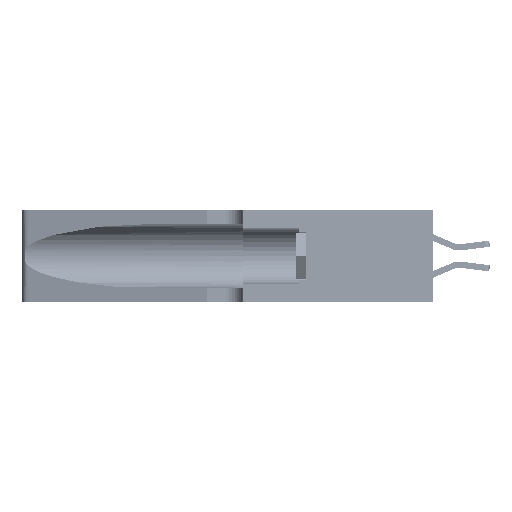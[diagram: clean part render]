
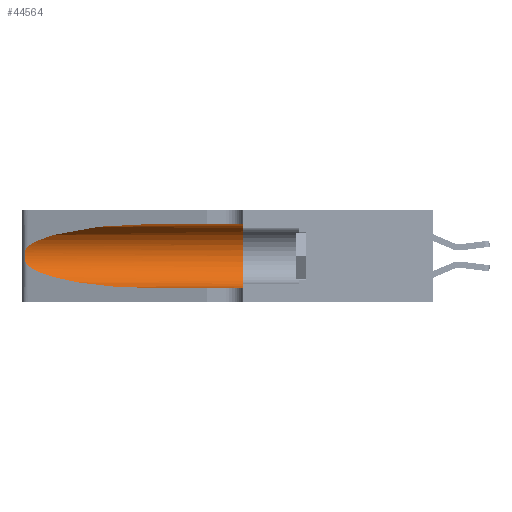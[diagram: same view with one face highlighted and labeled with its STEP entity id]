
A CAD part, left-side view. The second image highlights one B-rep face of the part: STEP entity #44564.
In plain terms, the highlighted cylindrical face has radius 3.308 mm (diameter 6.617 mm), a partial arc.
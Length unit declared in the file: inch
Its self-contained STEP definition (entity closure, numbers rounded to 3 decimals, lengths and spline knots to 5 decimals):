
#100 = EDGE_CURVE ( 'NONE', #24338, #21920, #4172, .T. ) ;
#194 = CARTESIAN_POINT ( 'NONE',  ( 0.18966, 0.96281, 0.31525 ) ) ;
#830 = CARTESIAN_POINT ( 'NONE',  ( 0.25487, 1.22718, 0.14631 ) ) ;
#2473 = CARTESIAN_POINT ( 'NONE',  ( 0.1305, 0.35, 0.185 ) ) ;
#3311 = EDGE_CURVE ( 'NONE', #43740, #45676, #7417, .T. ) ;
#3930 = CARTESIAN_POINT ( 'NONE',  ( 0.1305, 1.61858, 0.31525 ) ) ;
#4172 = LINE ( 'NONE', #41860, #13248 ) ;
#4499 = CARTESIAN_POINT ( 'NONE',  ( 0.26075, 1.23896, 0.19203 ) ) ;
#4829 = EDGE_CURVE ( 'NONE', #14940, #9047, #49689, .T. ) ;
#4967 =( BOUNDED_CURVE ( )  B_SPLINE_CURVE ( 3, ( #23889, #28094, #47500, #47327 ),
 .UNSPECIFIED., .F., .F. ) 
 B_SPLINE_CURVE_WITH_KNOTS ( ( 4, 4 ),
 ( 3.44316, 4.71239 ),
 .UNSPECIFIED. ) 
 CURVE ( )  GEOMETRIC_REPRESENTATION_ITEM ( )  RATIONAL_B_SPLINE_CURVE ( ( 1., 0.87, 0.87, 1. ) ) 
 REPRESENTATION_ITEM ( '' )  );
#5344 = CARTESIAN_POINT ( 'NONE',  ( 0.25487, 1.22718, 0.14631 ) ) ;
#5705 = CARTESIAN_POINT ( 'NONE',  ( 0.1305, 0.72297, 0.05475 ) ) ;
#7417 = B_SPLINE_CURVE_WITH_KNOTS ( 'NONE', 3,
 ( #39196, #27591, #23885, #12129, #42922, #46819, #4499, #31471, #23217, #35326, #19344, #20002, #46989, #830 ),
 .UNSPECIFIED., .F., .F.,
 ( 4, 2, 2, 2, 2, 2, 4 ),
 ( 0., 0.00027, 0.00053, 0.00107, 0.0016, 0.00187, 0.00214 ),
 .UNSPECIFIED. ) ;
#9047 = VERTEX_POINT ( 'NONE', #18773 ) ;
#9199 = DIRECTION ( 'NONE',  ( 0., -1., 0. ) ) ;
#12129 = CARTESIAN_POINT ( 'NONE',  ( 0.25787, 1.23484, 0.2124 ) ) ;
#13248 = VECTOR ( 'NONE', #9199, 39.37008 ) ;
#14940 = VERTEX_POINT ( 'NONE', #24426 ) ;
#16116 = EDGE_LOOP ( 'NONE', ( #29000, #22268, #26519, #30840, #21005, #29541 ) ) ;
#18773 = CARTESIAN_POINT ( 'NONE',  ( 0.1305, 0.35, 0.31525 ) ) ;
#19016 = CYLINDRICAL_SURFACE ( 'NONE', #40733, 0.13025 ) ;
#19344 = CARTESIAN_POINT ( 'NONE',  ( 0.25789, 1.23486, 0.15765 ) ) ;
#20002 = CARTESIAN_POINT ( 'NONE',  ( 0.25639, 1.23186, 0.15144 ) ) ;
#21005 = ORIENTED_EDGE ( 'NONE', *, *, #41717, .F. ) ;
#21920 = VERTEX_POINT ( 'NONE', #45777 ) ;
#22268 = ORIENTED_EDGE ( 'NONE', *, *, #3311, .T. ) ;
#23217 = CARTESIAN_POINT ( 'NONE',  ( 0.26017, 1.23833, 0.17102 ) ) ;
#23885 = CARTESIAN_POINT ( 'NONE',  ( 0.25639, 1.23184, 0.21858 ) ) ;
#23889 = CARTESIAN_POINT ( 'NONE',  ( 0.25487, 1.22718, 0.14631 ) ) ;
#24338 = VERTEX_POINT ( 'NONE', #5705 ) ;
#24426 = CARTESIAN_POINT ( 'NONE',  ( 0.1305, 0.72297, 0.31525 ) ) ;
#25877 = DIRECTION ( 'NONE',  ( 0., 0., -1. ) ) ;
#26519 = ORIENTED_EDGE ( 'NONE', *, *, #35315, .T. ) ;
#27591 = CARTESIAN_POINT ( 'NONE',  ( 0.25555, 1.22994, 0.2215 ) ) ;
#28094 = CARTESIAN_POINT ( 'NONE',  ( 0.2373, 1.15595, 0.08982 ) ) ;
#29000 = ORIENTED_EDGE ( 'NONE', *, *, #45574, .T. ) ;
#29541 = ORIENTED_EDGE ( 'NONE', *, *, #4829, .F. ) ;
#30840 = ORIENTED_EDGE ( 'NONE', *, *, #100, .T. ) ;
#31168 = CARTESIAN_POINT ( 'NONE',  ( 0.1305, 0.72297, 0.31525 ) ) ;
#31471 = CARTESIAN_POINT ( 'NONE',  ( 0.26075, 1.23896, 0.178 ) ) ;
#32400 = CIRCLE ( 'NONE', #44227, 0.13025 ) ;
#33436 = DIRECTION ( 'NONE',  ( 0., 0., 1. ) ) ;
#33958 = DIRECTION ( 'NONE',  ( 0., -1., 0. ) ) ;
#35315 = EDGE_CURVE ( 'NONE', #45676, #24338, #4967, .T. ) ;
#35326 = CARTESIAN_POINT ( 'NONE',  ( 0.25856, 1.23593, 0.16098 ) ) ;
#35541 = CARTESIAN_POINT ( 'NONE',  ( 0.25487, 1.22718, 0.22369 ) ) ;
#35797 = VECTOR ( 'NONE', #46400, 39.37008 ) ;
#39196 = CARTESIAN_POINT ( 'NONE',  ( 0.25487, 1.22718, 0.22369 ) ) ;
#40586 = CARTESIAN_POINT ( 'NONE',  ( 0.25487, 1.22718, 0.22369 ) ) ;
#40733 = AXIS2_PLACEMENT_3D ( 'NONE', #45420, #33958, #25877 ) ;
#41717 = EDGE_CURVE ( 'NONE', #9047, #21920, #32400, .T. ) ;
#41860 = CARTESIAN_POINT ( 'NONE',  ( 0.1305, 1.61858, 0.05475 ) ) ;
#42506 = FACE_OUTER_BOUND ( 'NONE', #16116, .T. ) ;
#42922 = CARTESIAN_POINT ( 'NONE',  ( 0.25854, 1.2359, 0.20912 ) ) ;
#43132 = CARTESIAN_POINT ( 'NONE',  ( 0.2373, 1.15595, 0.28018 ) ) ;
#43740 = VERTEX_POINT ( 'NONE', #40586 ) ;
#44227 = AXIS2_PLACEMENT_3D ( 'NONE', #2473, #44744, #33436 ) ;
#44564 = ADVANCED_FACE ( 'NONE', ( #42506 ), #19016, .F. ) ;
#44744 = DIRECTION ( 'NONE',  ( 0., 1., 0. ) ) ;
#45420 = CARTESIAN_POINT ( 'NONE',  ( 0.1305, 1.61858, 0.185 ) ) ;
#45574 = EDGE_CURVE ( 'NONE', #14940, #43740, #49149, .T. ) ;
#45676 = VERTEX_POINT ( 'NONE', #5344 ) ;
#45777 = CARTESIAN_POINT ( 'NONE',  ( 0.1305, 0.35, 0.05475 ) ) ;
#46400 = DIRECTION ( 'NONE',  ( 0., -1., 0. ) ) ;
#46819 = CARTESIAN_POINT ( 'NONE',  ( 0.26018, 1.23835, 0.19895 ) ) ;
#46989 = CARTESIAN_POINT ( 'NONE',  ( 0.25555, 1.22993, 0.14849 ) ) ;
#47327 = CARTESIAN_POINT ( 'NONE',  ( 0.1305, 0.72297, 0.05475 ) ) ;
#47500 = CARTESIAN_POINT ( 'NONE',  ( 0.18966, 0.96281, 0.05475 ) ) ;
#49149 =( BOUNDED_CURVE ( )  B_SPLINE_CURVE ( 3, ( #31168, #194, #43132, #35541 ),
 .UNSPECIFIED., .F., .F. ) 
 B_SPLINE_CURVE_WITH_KNOTS ( ( 4, 4 ),
 ( 1.5708, 2.84003 ),
 .UNSPECIFIED. ) 
 CURVE ( )  GEOMETRIC_REPRESENTATION_ITEM ( )  RATIONAL_B_SPLINE_CURVE ( ( 1., 0.87, 0.87, 1. ) ) 
 REPRESENTATION_ITEM ( '' )  );
#49689 = LINE ( 'NONE', #3930, #35797 ) ;
